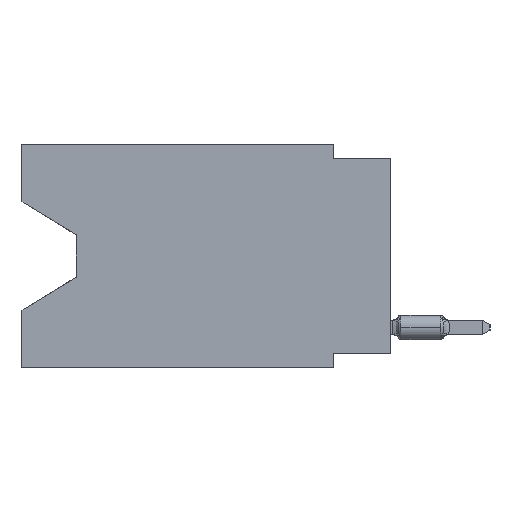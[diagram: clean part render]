
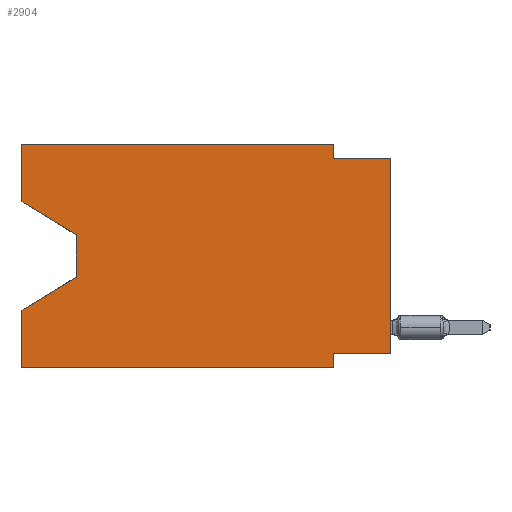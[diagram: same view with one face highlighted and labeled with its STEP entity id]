
A CAD part, left-side view. The second image highlights one B-rep face of the part: STEP entity #2904.
In plain terms, the highlighted planar face has unit normal (-1, 0, 0).
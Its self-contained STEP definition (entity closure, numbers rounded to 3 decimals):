
#303 = ORIENTED_EDGE ( 'NONE', *, *, #73312, .T. ) ;
#689 = CARTESIAN_POINT ( 'NONE',  ( 0., 16.383, 0. ) ) ;
#2904 = ADVANCED_FACE ( 'NONE', ( #45785 ), #33025, .F. ) ;
#3488 = EDGE_CURVE ( 'NONE', #28204, #38059, #36631, .T. ) ;
#3854 = CARTESIAN_POINT ( 'NONE',  ( 0., 16.383, 0. ) ) ;
#4154 = LINE ( 'NONE', #10119, #17796 ) ;
#4312 = AXIS2_PLACEMENT_3D ( 'NONE', #13500, #33449, #59775 ) ;
#4792 = VERTEX_POINT ( 'NONE', #52959 ) ;
#5806 = LINE ( 'NONE', #76757, #60102 ) ;
#6863 = VECTOR ( 'NONE', #19770, 1000. ) ;
#8206 = CARTESIAN_POINT ( 'NONE',  ( 0., 16.383, -9.906 ) ) ;
#8968 = ORIENTED_EDGE ( 'NONE', *, *, #53178, .F. ) ;
#10119 = CARTESIAN_POINT ( 'NONE',  ( 0., 16.383, -2.546 ) ) ;
#10896 = DIRECTION ( 'NONE',  ( 0., -1., 0. ) ) ;
#11058 = CARTESIAN_POINT ( 'NONE',  ( 0., 2.54, 0. ) ) ;
#11964 = CARTESIAN_POINT ( 'NONE',  ( 0., 16.383, -7.36 ) ) ;
#13082 = VERTEX_POINT ( 'NONE', #34442 ) ;
#13500 = CARTESIAN_POINT ( 'NONE',  ( 0., 16.383, 0. ) ) ;
#15570 = EDGE_CURVE ( 'NONE', #4792, #68532, #64211, .T. ) ;
#15674 = EDGE_CURVE ( 'NONE', #51101, #22232, #33164, .T. ) ;
#17796 = VECTOR ( 'NONE', #82331, 1000. ) ;
#17897 = CARTESIAN_POINT ( 'NONE',  ( 0., 0., 0. ) ) ;
#18526 = CARTESIAN_POINT ( 'NONE',  ( 0., 0., -0.635 ) ) ;
#18800 = CARTESIAN_POINT ( 'NONE',  ( 0., 16.383, 0. ) ) ;
#19478 = DIRECTION ( 'NONE',  ( 0., 1., 0. ) ) ;
#19770 = DIRECTION ( 'NONE',  ( 0., 0., 1. ) ) ;
#20017 = ORIENTED_EDGE ( 'NONE', *, *, #40363, .F. ) ;
#20208 = VECTOR ( 'NONE', #23390, 1000. ) ;
#20534 = CARTESIAN_POINT ( 'NONE',  ( 0., 2.54, -9.906 ) ) ;
#20595 = VECTOR ( 'NONE', #25533, 1000. ) ;
#20633 = CARTESIAN_POINT ( 'NONE',  ( 0., 2.54, -9.906 ) ) ;
#22232 = VERTEX_POINT ( 'NONE', #62654 ) ;
#23390 = DIRECTION ( 'NONE',  ( 0., -1., 0. ) ) ;
#23811 = LINE ( 'NONE', #3854, #20208 ) ;
#25533 = DIRECTION ( 'NONE',  ( 0., 0., -1. ) ) ;
#25751 = DIRECTION ( 'NONE',  ( 0., 0.855, -0.519 ) ) ;
#26047 = VECTOR ( 'NONE', #37861, 1000. ) ;
#26794 = CARTESIAN_POINT ( 'NONE',  ( 0., 2.54, 0. ) ) ;
#27273 = EDGE_CURVE ( 'NONE', #4792, #13082, #70284, .T. ) ;
#27766 = ORIENTED_EDGE ( 'NONE', *, *, #15570, .T. ) ;
#28204 = VERTEX_POINT ( 'NONE', #8206 ) ;
#30253 = CARTESIAN_POINT ( 'NONE',  ( 0., 16.383, -9.906 ) ) ;
#31693 = LINE ( 'NONE', #18526, #37977 ) ;
#32388 = VERTEX_POINT ( 'NONE', #62406 ) ;
#33025 = PLANE ( 'NONE',  #4312 ) ;
#33164 = LINE ( 'NONE', #26794, #36897 ) ;
#33449 = DIRECTION ( 'NONE',  ( 1., 0., 0. ) ) ;
#33848 = ORIENTED_EDGE ( 'NONE', *, *, #61542, .T. ) ;
#34169 = CARTESIAN_POINT ( 'NONE',  ( 0., 0., -0.635 ) ) ;
#34442 = CARTESIAN_POINT ( 'NONE',  ( 0., 2.54, -9.271 ) ) ;
#36631 = LINE ( 'NONE', #30253, #80588 ) ;
#36897 = VECTOR ( 'NONE', #39537, 1000. ) ;
#37552 = EDGE_CURVE ( 'NONE', #32388, #77498, #5806, .T. ) ;
#37861 = DIRECTION ( 'NONE',  ( 0., 0., 1. ) ) ;
#37977 = VECTOR ( 'NONE', #10896, 1000. ) ;
#38059 = VERTEX_POINT ( 'NONE', #20534 ) ;
#38935 = EDGE_CURVE ( 'NONE', #22232, #68532, #31693, .T. ) ;
#39537 = DIRECTION ( 'NONE',  ( 0., 0., -1. ) ) ;
#40363 = EDGE_CURVE ( 'NONE', #13082, #38059, #78843, .T. ) ;
#42608 = CARTESIAN_POINT ( 'NONE',  ( 0., 16.383, -2.546 ) ) ;
#44603 = VERTEX_POINT ( 'NONE', #53940 ) ;
#45308 = DIRECTION ( 'NONE',  ( 0., 0., 1. ) ) ;
#45726 = LINE ( 'NONE', #689, #83216 ) ;
#45785 = FACE_OUTER_BOUND ( 'NONE', #67832, .T. ) ;
#46366 = DIRECTION ( 'NONE',  ( 0., -1., 0. ) ) ;
#46538 = DIRECTION ( 'NONE',  ( 0., 0., -1. ) ) ;
#46623 = ORIENTED_EDGE ( 'NONE', *, *, #37552, .T. ) ;
#46829 = VECTOR ( 'NONE', #19478, 1000. ) ;
#48687 = VECTOR ( 'NONE', #46538, 1000. ) ;
#51101 = VERTEX_POINT ( 'NONE', #11058 ) ;
#52959 = CARTESIAN_POINT ( 'NONE',  ( 0., 0., -9.271 ) ) ;
#53178 = EDGE_CURVE ( 'NONE', #28204, #77498, #64396, .T. ) ;
#53940 = CARTESIAN_POINT ( 'NONE',  ( 0., 13.97, -4.013 ) ) ;
#55866 = ORIENTED_EDGE ( 'NONE', *, *, #38935, .F. ) ;
#59079 = CARTESIAN_POINT ( 'NONE',  ( 0., 13.97, -4.013 ) ) ;
#59490 = LINE ( 'NONE', #59079, #20595 ) ;
#59775 = DIRECTION ( 'NONE',  ( 0., 0., -1. ) ) ;
#59984 = ORIENTED_EDGE ( 'NONE', *, *, #71787, .F. ) ;
#60102 = VECTOR ( 'NONE', #25751, 1000. ) ;
#61542 = EDGE_CURVE ( 'NONE', #44603, #32388, #59490, .T. ) ;
#61861 = ORIENTED_EDGE ( 'NONE', *, *, #15674, .F. ) ;
#62406 = CARTESIAN_POINT ( 'NONE',  ( 0., 13.97, -5.893 ) ) ;
#62654 = CARTESIAN_POINT ( 'NONE',  ( 0., 2.54, -0.635 ) ) ;
#64211 = LINE ( 'NONE', #17897, #26047 ) ;
#64396 = LINE ( 'NONE', #65227, #6863 ) ;
#65227 = CARTESIAN_POINT ( 'NONE',  ( 0., 16.383, 0. ) ) ;
#67279 = VERTEX_POINT ( 'NONE', #18800 ) ;
#67411 = ORIENTED_EDGE ( 'NONE', *, *, #3488, .T. ) ;
#67832 = EDGE_LOOP ( 'NONE', ( #303, #33848, #46623, #8968, #67411, #20017, #76289, #27766, #55866, #61861, #59984, #75515 ) ) ;
#68532 = VERTEX_POINT ( 'NONE', #34169 ) ;
#70284 = LINE ( 'NONE', #77689, #46829 ) ;
#71787 = EDGE_CURVE ( 'NONE', #67279, #51101, #23811, .T. ) ;
#73312 = EDGE_CURVE ( 'NONE', #79793, #44603, #4154, .T. ) ;
#75515 = ORIENTED_EDGE ( 'NONE', *, *, #77920, .F. ) ;
#76289 = ORIENTED_EDGE ( 'NONE', *, *, #27273, .F. ) ;
#76757 = CARTESIAN_POINT ( 'NONE',  ( 0., 13.97, -5.893 ) ) ;
#77498 = VERTEX_POINT ( 'NONE', #11964 ) ;
#77689 = CARTESIAN_POINT ( 'NONE',  ( 0., 0., -9.271 ) ) ;
#77920 = EDGE_CURVE ( 'NONE', #79793, #67279, #45726, .T. ) ;
#78843 = LINE ( 'NONE', #20633, #48687 ) ;
#79793 = VERTEX_POINT ( 'NONE', #42608 ) ;
#80588 = VECTOR ( 'NONE', #46366, 1000. ) ;
#82331 = DIRECTION ( 'NONE',  ( 0., -0.855, -0.519 ) ) ;
#83216 = VECTOR ( 'NONE', #45308, 1000. ) ;
